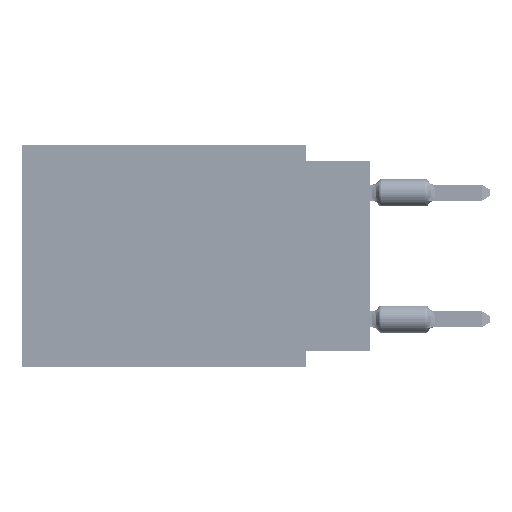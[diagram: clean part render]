
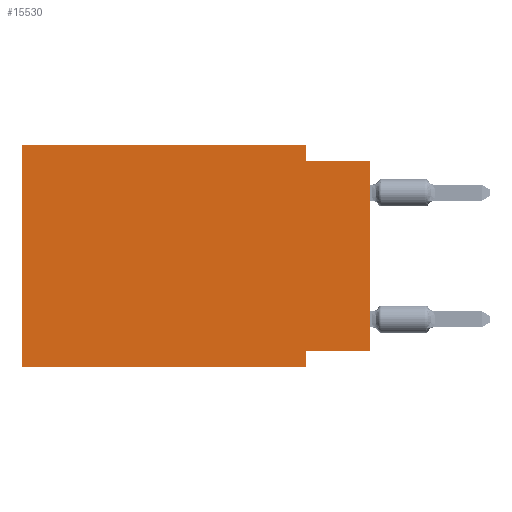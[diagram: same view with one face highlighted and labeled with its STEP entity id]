
A CAD part, left-side view. The second image highlights one B-rep face of the part: STEP entity #15530.
In plain terms, the highlighted planar face has unit normal (-1, 0, 0).
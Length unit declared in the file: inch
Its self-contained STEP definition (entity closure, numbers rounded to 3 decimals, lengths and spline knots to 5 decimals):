
#758 = EDGE_CURVE ( 'NONE', #47640, #69894, #16568, .T. ) ;
#2160 = LINE ( 'NONE', #22916, #60690 ) ;
#2448 = VERTEX_POINT ( 'NONE', #39452 ) ;
#3466 = DIRECTION ( 'NONE',  ( 0., 0., -1. ) ) ;
#3806 = CARTESIAN_POINT ( 'NONE',  ( 0., 0.55, -0.35 ) ) ;
#4460 = VECTOR ( 'NONE', #57137, 39.37008 ) ;
#7719 = ORIENTED_EDGE ( 'NONE', *, *, #53897, .F. ) ;
#8073 = LINE ( 'NONE', #28341, #40808 ) ;
#8594 = CARTESIAN_POINT ( 'NONE',  ( 0., 0.55, 0. ) ) ;
#9318 = LINE ( 'NONE', #84242, #4460 ) ;
#9804 = CARTESIAN_POINT ( 'NONE',  ( 0., 0.1, -0.35 ) ) ;
#11210 = CARTESIAN_POINT ( 'NONE',  ( 0., 0.55, 0. ) ) ;
#13278 = DIRECTION ( 'NONE',  ( 0., -1., 0. ) ) ;
#15530 = ADVANCED_FACE ( 'NONE', ( #77632 ), #22999, .F. ) ;
#16551 = VECTOR ( 'NONE', #23564, 39.37008 ) ;
#16568 = LINE ( 'NONE', #42747, #56444 ) ;
#16735 = CARTESIAN_POINT ( 'NONE',  ( 0., 0., -0.025 ) ) ;
#20846 = CARTESIAN_POINT ( 'NONE',  ( 0., 0., -0.325 ) ) ;
#22916 = CARTESIAN_POINT ( 'NONE',  ( 0., 0.1, 0. ) ) ;
#22999 = PLANE ( 'NONE',  #84543 ) ;
#23115 = CARTESIAN_POINT ( 'NONE',  ( 0., 0., 0. ) ) ;
#23564 = DIRECTION ( 'NONE',  ( 0., 0., 1. ) ) ;
#23708 = ORIENTED_EDGE ( 'NONE', *, *, #59991, .T. ) ;
#25128 = VERTEX_POINT ( 'NONE', #20846 ) ;
#25248 = VECTOR ( 'NONE', #66186, 39.37008 ) ;
#25334 = CARTESIAN_POINT ( 'NONE',  ( 0., 0.1, -0.325 ) ) ;
#26485 = VERTEX_POINT ( 'NONE', #16735 ) ;
#28341 = CARTESIAN_POINT ( 'NONE',  ( 0., 0., -0.025 ) ) ;
#29670 = DIRECTION ( 'NONE',  ( 0., 0., -1. ) ) ;
#33115 = CARTESIAN_POINT ( 'NONE',  ( 0., 0.55, 0. ) ) ;
#37403 = DIRECTION ( 'NONE',  ( 1., 0., 0. ) ) ;
#37642 = DIRECTION ( 'NONE',  ( 0., -1., 0. ) ) ;
#39452 = CARTESIAN_POINT ( 'NONE',  ( 0., 0.1, 0. ) ) ;
#40808 = VECTOR ( 'NONE', #55883, 39.37008 ) ;
#42747 = CARTESIAN_POINT ( 'NONE',  ( 0., 0.1, -0.35 ) ) ;
#42856 = LINE ( 'NONE', #86506, #25248 ) ;
#43859 = ORIENTED_EDGE ( 'NONE', *, *, #60491, .F. ) ;
#44419 = LINE ( 'NONE', #3806, #69679 ) ;
#46008 = ORIENTED_EDGE ( 'NONE', *, *, #56497, .T. ) ;
#47640 = VERTEX_POINT ( 'NONE', #25334 ) ;
#47740 = ORIENTED_EDGE ( 'NONE', *, *, #87724, .F. ) ;
#48343 = ORIENTED_EDGE ( 'NONE', *, *, #66920, .F. ) ;
#50536 = VERTEX_POINT ( 'NONE', #75374 ) ;
#51517 = LINE ( 'NONE', #23115, #16551 ) ;
#53897 = EDGE_CURVE ( 'NONE', #56715, #78960, #9318, .T. ) ;
#54031 = VECTOR ( 'NONE', #13278, 39.37008 ) ;
#55883 = DIRECTION ( 'NONE',  ( 0., -1., 0. ) ) ;
#56444 = VECTOR ( 'NONE', #3466, 39.37008 ) ;
#56497 = EDGE_CURVE ( 'NONE', #56715, #69894, #44419, .T. ) ;
#56715 = VERTEX_POINT ( 'NONE', #75993 ) ;
#57137 = DIRECTION ( 'NONE',  ( 0., 0., 1. ) ) ;
#57914 = ORIENTED_EDGE ( 'NONE', *, *, #758, .F. ) ;
#59991 = EDGE_CURVE ( 'NONE', #25128, #26485, #51517, .T. ) ;
#60491 = EDGE_CURVE ( 'NONE', #25128, #47640, #42856, .T. ) ;
#60690 = VECTOR ( 'NONE', #29670, 39.37008 ) ;
#66186 = DIRECTION ( 'NONE',  ( 0., 1., 0. ) ) ;
#66920 = EDGE_CURVE ( 'NONE', #50536, #26485, #8073, .T. ) ;
#69679 = VECTOR ( 'NONE', #37642, 39.37008 ) ;
#69894 = VERTEX_POINT ( 'NONE', #9804 ) ;
#75374 = CARTESIAN_POINT ( 'NONE',  ( 0., 0.1, -0.025 ) ) ;
#75993 = CARTESIAN_POINT ( 'NONE',  ( 0., 0.55, -0.35 ) ) ;
#76722 = ORIENTED_EDGE ( 'NONE', *, *, #80480, .F. ) ;
#77632 = FACE_OUTER_BOUND ( 'NONE', #83845, .T. ) ;
#78960 = VERTEX_POINT ( 'NONE', #11210 ) ;
#80480 = EDGE_CURVE ( 'NONE', #78960, #2448, #80992, .T. ) ;
#80992 = LINE ( 'NONE', #33115, #54031 ) ;
#83516 = DIRECTION ( 'NONE',  ( 0., 0., -1. ) ) ;
#83845 = EDGE_LOOP ( 'NONE', ( #23708, #48343, #47740, #76722, #7719, #46008, #57914, #43859 ) ) ;
#84242 = CARTESIAN_POINT ( 'NONE',  ( 0., 0.55, 0. ) ) ;
#84543 = AXIS2_PLACEMENT_3D ( 'NONE', #8594, #37403, #83516 ) ;
#86506 = CARTESIAN_POINT ( 'NONE',  ( 0., 0., -0.325 ) ) ;
#87724 = EDGE_CURVE ( 'NONE', #2448, #50536, #2160, .T. ) ;
